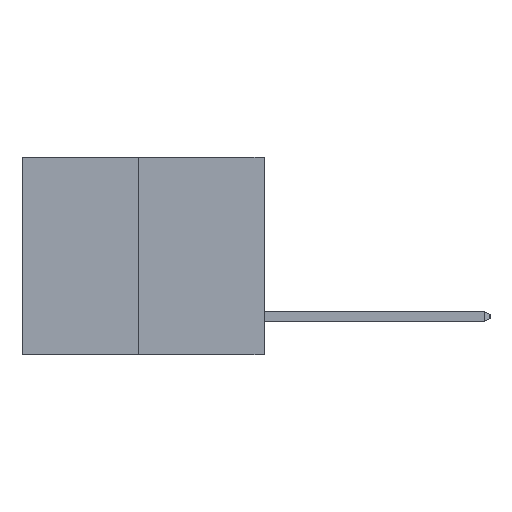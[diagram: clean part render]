
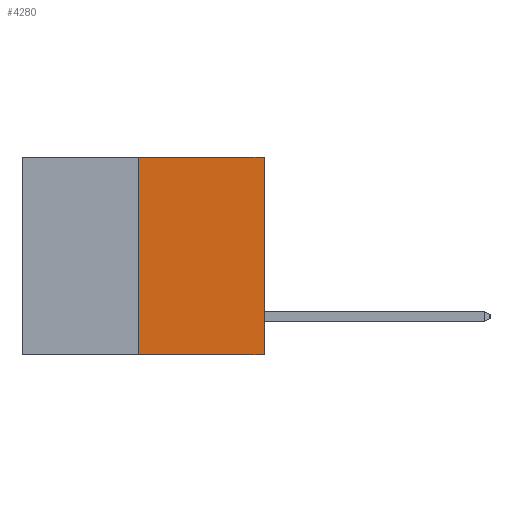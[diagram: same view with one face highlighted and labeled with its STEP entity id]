
A CAD part, left-side view. The second image highlights one B-rep face of the part: STEP entity #4280.
In plain terms, the highlighted planar face has unit normal (-1, 0, 0).
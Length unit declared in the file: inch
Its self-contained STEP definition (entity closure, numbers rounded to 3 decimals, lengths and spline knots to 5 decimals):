
#670 = CARTESIAN_POINT ( 'NONE',  ( 0., 0.6, 0. ) ) ;
#761 = EDGE_CURVE ( 'NONE', #3342, #13329, #19972, .T. ) ;
#903 = CARTESIAN_POINT ( 'NONE',  ( 0., 0.312, -0.49 ) ) ;
#1021 = VECTOR ( 'NONE', #6598, 39.37008 ) ;
#1365 = EDGE_CURVE ( 'NONE', #13329, #11271, #3327, .T. ) ;
#1467 = EDGE_LOOP ( 'NONE', ( #13247, #11865, #17338, #1801 ) ) ;
#1801 = ORIENTED_EDGE ( 'NONE', *, *, #1365, .F. ) ;
#1962 = CARTESIAN_POINT ( 'NONE',  ( 0., 0.6, -0.49 ) ) ;
#2399 = VECTOR ( 'NONE', #5723, 39.37008 ) ;
#2428 = EDGE_CURVE ( 'NONE', #3342, #17781, #15238, .T. ) ;
#2443 = DIRECTION ( 'NONE',  ( 0., 0., 1. ) ) ;
#2572 = VECTOR ( 'NONE', #2443, 39.37008 ) ;
#2581 = CARTESIAN_POINT ( 'NONE',  ( 0., 0., 0. ) ) ;
#3327 = LINE ( 'NONE', #670, #8929 ) ;
#3342 = VERTEX_POINT ( 'NONE', #12842 ) ;
#4280 = ADVANCED_FACE ( 'NONE', ( #8306 ), #5145, .F. ) ;
#4951 = CARTESIAN_POINT ( 'NONE',  ( 0., 0.6, 0. ) ) ;
#5145 = PLANE ( 'NONE',  #17270 ) ;
#5723 = DIRECTION ( 'NONE',  ( 0., 0., 1. ) ) ;
#6598 = DIRECTION ( 'NONE',  ( 0., -1., 0. ) ) ;
#6725 = DIRECTION ( 'NONE',  ( 0., 0., -1. ) ) ;
#8306 = FACE_OUTER_BOUND ( 'NONE', #1467, .T. ) ;
#8929 = VECTOR ( 'NONE', #18651, 39.37008 ) ;
#9422 = LINE ( 'NONE', #2581, #2572 ) ;
#10631 = CARTESIAN_POINT ( 'NONE',  ( 0., 0.312, 0. ) ) ;
#11271 = VERTEX_POINT ( 'NONE', #18956 ) ;
#11329 = EDGE_CURVE ( 'NONE', #17781, #11271, #9422, .T. ) ;
#11865 = ORIENTED_EDGE ( 'NONE', *, *, #2428, .T. ) ;
#12842 = CARTESIAN_POINT ( 'NONE',  ( 0., 0.312, -0.49 ) ) ;
#13247 = ORIENTED_EDGE ( 'NONE', *, *, #761, .F. ) ;
#13329 = VERTEX_POINT ( 'NONE', #10631 ) ;
#15238 = LINE ( 'NONE', #1962, #1021 ) ;
#16528 = DIRECTION ( 'NONE',  ( 1., 0., 0. ) ) ;
#17270 = AXIS2_PLACEMENT_3D ( 'NONE', #4951, #16528, #6725 ) ;
#17338 = ORIENTED_EDGE ( 'NONE', *, *, #11329, .T. ) ;
#17781 = VERTEX_POINT ( 'NONE', #17901 ) ;
#17901 = CARTESIAN_POINT ( 'NONE',  ( 0., 0., -0.49 ) ) ;
#18651 = DIRECTION ( 'NONE',  ( 0., -1., 0. ) ) ;
#18956 = CARTESIAN_POINT ( 'NONE',  ( 0., 0., 0. ) ) ;
#19972 = LINE ( 'NONE', #903, #2399 ) ;
